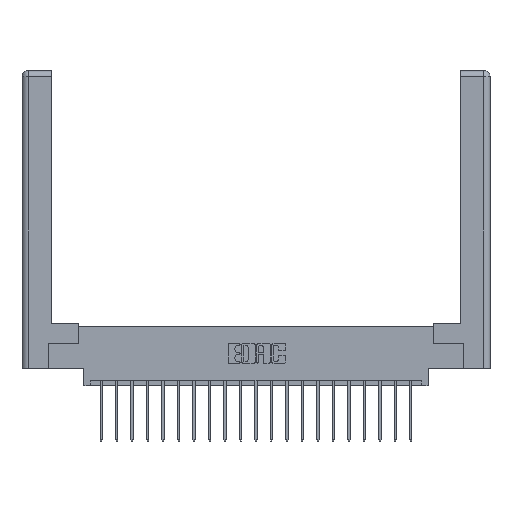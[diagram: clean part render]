
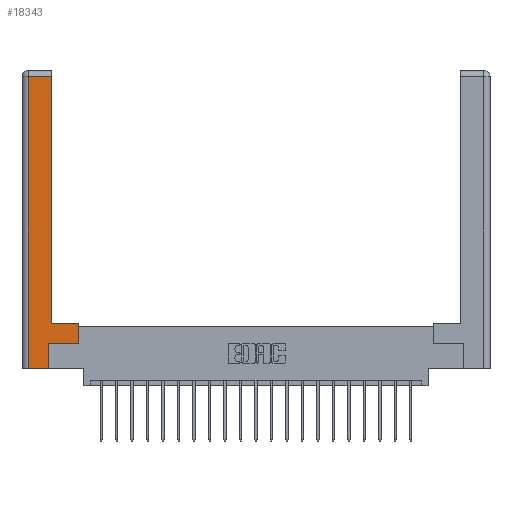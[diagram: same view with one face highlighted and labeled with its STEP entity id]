
A CAD part, top view. The second image highlights one B-rep face of the part: STEP entity #18343.
In plain terms, the highlighted planar face has unit normal (0, 0, 1).
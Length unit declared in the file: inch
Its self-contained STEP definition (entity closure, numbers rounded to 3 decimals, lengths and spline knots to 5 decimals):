
#148 = VERTEX_POINT ( 'NONE', #16869 ) ;
#1319 = CARTESIAN_POINT ( 'NONE',  ( 0.0615, 0., 0. ) ) ;
#1491 = VECTOR ( 'NONE', #8864, 39.37008 ) ;
#1830 = DIRECTION ( 'NONE',  ( 0., 0., -1. ) ) ;
#1942 = VECTOR ( 'NONE', #8019, 39.37008 ) ;
#1955 = CARTESIAN_POINT ( 'NONE',  ( 0.0615, 2.94, 0. ) ) ;
#2761 = EDGE_LOOP ( 'NONE', ( #13976, #9997, #12916, #21723, #21658, #9606, #14345, #12355 ) ) ;
#2775 = EDGE_CURVE ( 'NONE', #8805, #148, #10403, .T. ) ;
#3117 = EDGE_CURVE ( 'NONE', #21715, #8658, #19420, .T. ) ;
#3564 = PLANE ( 'NONE',  #9923 ) ;
#3602 = CARTESIAN_POINT ( 'NONE',  ( 0.0615, 0., 0. ) ) ;
#3996 = LINE ( 'NONE', #3602, #8477 ) ;
#4587 = EDGE_CURVE ( 'NONE', #11776, #8805, #9748, .T. ) ;
#4599 = DIRECTION ( 'NONE',  ( 0., 1., 0. ) ) ;
#4836 = DIRECTION ( 'NONE',  ( 1., 0., 0. ) ) ;
#4883 = LINE ( 'NONE', #14941, #5929 ) ;
#5929 = VECTOR ( 'NONE', #4836, 39.37008 ) ;
#7064 = DIRECTION ( 'NONE',  ( -1., 0., 0. ) ) ;
#7071 = VERTEX_POINT ( 'NONE', #12902 ) ;
#7204 = EDGE_CURVE ( 'NONE', #148, #16820, #3996, .T. ) ;
#7275 = CARTESIAN_POINT ( 'NONE',  ( 0.265, 0.245, 0. ) ) ;
#7561 = CARTESIAN_POINT ( 'NONE',  ( 0.565, 0.45, 0. ) ) ;
#7814 = FACE_OUTER_BOUND ( 'NONE', #2761, .T. ) ;
#8019 = DIRECTION ( 'NONE',  ( 0., 1., 0. ) ) ;
#8477 = VECTOR ( 'NONE', #20062, 39.37008 ) ;
#8658 = VERTEX_POINT ( 'NONE', #15937 ) ;
#8805 = VERTEX_POINT ( 'NONE', #14947 ) ;
#8864 = DIRECTION ( 'NONE',  ( -1., 0., 0. ) ) ;
#9606 = ORIENTED_EDGE ( 'NONE', *, *, #3117, .T. ) ;
#9748 = LINE ( 'NONE', #13177, #13674 ) ;
#9923 = AXIS2_PLACEMENT_3D ( 'NONE', #16986, #1830, #7064 ) ;
#9997 = ORIENTED_EDGE ( 'NONE', *, *, #2775, .T. ) ;
#10196 = LINE ( 'NONE', #14416, #16509 ) ;
#10295 = EDGE_CURVE ( 'NONE', #7071, #21715, #10196, .T. ) ;
#10403 = LINE ( 'NONE', #1955, #1491 ) ;
#11776 = VERTEX_POINT ( 'NONE', #21066 ) ;
#12355 = ORIENTED_EDGE ( 'NONE', *, *, #16998, .T. ) ;
#12902 = CARTESIAN_POINT ( 'NONE',  ( 0.265, 0., 0. ) ) ;
#12916 = ORIENTED_EDGE ( 'NONE', *, *, #7204, .T. ) ;
#13177 = CARTESIAN_POINT ( 'NONE',  ( 0.295, 3., 0. ) ) ;
#13674 = VECTOR ( 'NONE', #15655, 39.37008 ) ;
#13711 = CARTESIAN_POINT ( 'NONE',  ( 0.295, 0.45, 0. ) ) ;
#13976 = ORIENTED_EDGE ( 'NONE', *, *, #4587, .T. ) ;
#14345 = ORIENTED_EDGE ( 'NONE', *, *, #20924, .T. ) ;
#14416 = CARTESIAN_POINT ( 'NONE',  ( 0.265, 0.245, 0. ) ) ;
#14885 = VECTOR ( 'NONE', #18777, 39.37008 ) ;
#14941 = CARTESIAN_POINT ( 'NONE',  ( 0.265, 0., 0. ) ) ;
#14947 = CARTESIAN_POINT ( 'NONE',  ( 0.295, 2.94, 0. ) ) ;
#15270 = CARTESIAN_POINT ( 'NONE',  ( 0.565, 0.245, 0. ) ) ;
#15406 = DIRECTION ( 'NONE',  ( -1., 0., 0. ) ) ;
#15655 = DIRECTION ( 'NONE',  ( 0., 1., 0. ) ) ;
#15937 = CARTESIAN_POINT ( 'NONE',  ( 0.565, 0.245, 0. ) ) ;
#16509 = VECTOR ( 'NONE', #4599, 39.37008 ) ;
#16820 = VERTEX_POINT ( 'NONE', #1319 ) ;
#16869 = CARTESIAN_POINT ( 'NONE',  ( 0.0615, 2.94, 0. ) ) ;
#16986 = CARTESIAN_POINT ( 'NONE',  ( 0., 0., 0. ) ) ;
#16998 = EDGE_CURVE ( 'NONE', #18847, #11776, #21705, .T. ) ;
#18343 = ADVANCED_FACE ( 'NONE', ( #7814 ), #3564, .F. ) ;
#18777 = DIRECTION ( 'NONE',  ( 1., 0., 0. ) ) ;
#18847 = VERTEX_POINT ( 'NONE', #7561 ) ;
#19333 = LINE ( 'NONE', #21508, #1942 ) ;
#19420 = LINE ( 'NONE', #15270, #14885 ) ;
#19977 = EDGE_CURVE ( 'NONE', #16820, #7071, #4883, .T. ) ;
#20062 = DIRECTION ( 'NONE',  ( 0., -1., 0. ) ) ;
#20659 = VECTOR ( 'NONE', #15406, 39.37008 ) ;
#20924 = EDGE_CURVE ( 'NONE', #8658, #18847, #19333, .T. ) ;
#21066 = CARTESIAN_POINT ( 'NONE',  ( 0.295, 0.45, 0. ) ) ;
#21508 = CARTESIAN_POINT ( 'NONE',  ( 0.565, 0.45, 0. ) ) ;
#21658 = ORIENTED_EDGE ( 'NONE', *, *, #10295, .T. ) ;
#21705 = LINE ( 'NONE', #13711, #20659 ) ;
#21715 = VERTEX_POINT ( 'NONE', #7275 ) ;
#21723 = ORIENTED_EDGE ( 'NONE', *, *, #19977, .T. ) ;
